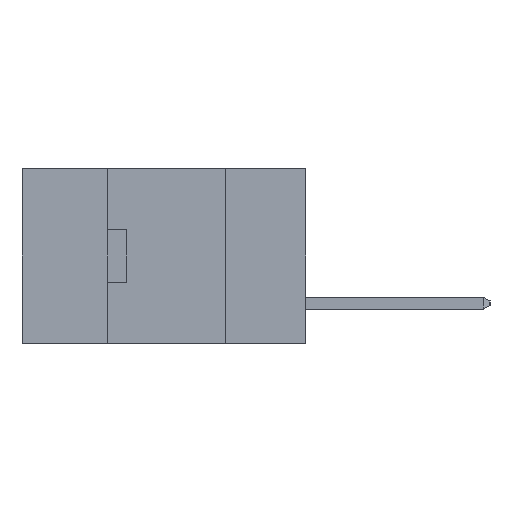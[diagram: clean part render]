
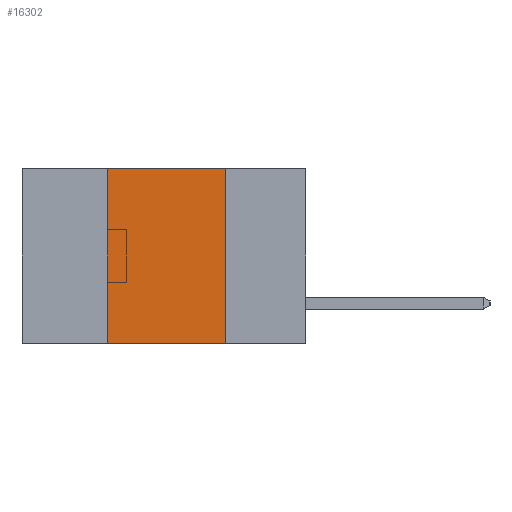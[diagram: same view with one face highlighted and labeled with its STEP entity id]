
A CAD part, left-side view. The second image highlights one B-rep face of the part: STEP entity #16302.
In plain terms, the highlighted planar face has unit normal (-1, 0, 0).
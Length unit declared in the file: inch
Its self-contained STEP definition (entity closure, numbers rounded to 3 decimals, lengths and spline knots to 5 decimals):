
#242 = ORIENTED_EDGE ( 'NONE', *, *, #8202, .F. ) ;
#1352 = PLANE ( 'NONE',  #19787 ) ;
#1804 = CARTESIAN_POINT ( 'NONE',  ( 0., 0.17, -0.37 ) ) ;
#2354 = VECTOR ( 'NONE', #24073, 39.37008 ) ;
#3273 = EDGE_CURVE ( 'NONE', #8465, #3703, #25556, .T. ) ;
#3518 = VERTEX_POINT ( 'NONE', #4085 ) ;
#3623 = DIRECTION ( 'NONE',  ( 0., 0., -1. ) ) ;
#3703 = VERTEX_POINT ( 'NONE', #25374 ) ;
#4085 = CARTESIAN_POINT ( 'NONE',  ( 0., 0.17, 0. ) ) ;
#4532 = VECTOR ( 'NONE', #14886, 39.37008 ) ;
#5842 = ORIENTED_EDGE ( 'NONE', *, *, #13503, .T. ) ;
#7167 = EDGE_LOOP ( 'NONE', ( #242, #24937, #26208, #5842 ) ) ;
#7629 = VECTOR ( 'NONE', #22485, 39.37008 ) ;
#7667 = CARTESIAN_POINT ( 'NONE',  ( 0., 0.6, 0. ) ) ;
#8202 = EDGE_CURVE ( 'NONE', #3518, #15794, #16063, .T. ) ;
#8465 = VERTEX_POINT ( 'NONE', #21970 ) ;
#10513 = CARTESIAN_POINT ( 'NONE',  ( 0., 0.17, -0.37 ) ) ;
#13503 = EDGE_CURVE ( 'NONE', #8465, #15794, #14542, .T. ) ;
#14542 = LINE ( 'NONE', #22995, #19451 ) ;
#14760 = DIRECTION ( 'NONE',  ( 0., -1., 0. ) ) ;
#14886 = DIRECTION ( 'NONE',  ( 0., 0., -1. ) ) ;
#15061 = FACE_OUTER_BOUND ( 'NONE', #7167, .T. ) ;
#15794 = VERTEX_POINT ( 'NONE', #10513 ) ;
#16063 = LINE ( 'NONE', #1804, #4532 ) ;
#16302 = ADVANCED_FACE ( 'NONE', ( #15061 ), #1352, .F. ) ;
#16573 = DIRECTION ( 'NONE',  ( 1., 0., 0. ) ) ;
#19451 = VECTOR ( 'NONE', #14760, 39.37008 ) ;
#19787 = AXIS2_PLACEMENT_3D ( 'NONE', #22699, #16573, #3623 ) ;
#21033 = EDGE_CURVE ( 'NONE', #3703, #3518, #23153, .T. ) ;
#21970 = CARTESIAN_POINT ( 'NONE',  ( 0., 0.42, -0.37 ) ) ;
#22485 = DIRECTION ( 'NONE',  ( 0., -1., 0. ) ) ;
#22699 = CARTESIAN_POINT ( 'NONE',  ( 0., 0.6, 0. ) ) ;
#22995 = CARTESIAN_POINT ( 'NONE',  ( 0., 0.6, -0.37 ) ) ;
#23153 = LINE ( 'NONE', #7667, #7629 ) ;
#24073 = DIRECTION ( 'NONE',  ( 0., 0., 1. ) ) ;
#24507 = CARTESIAN_POINT ( 'NONE',  ( 0., 0.42, -0.37 ) ) ;
#24937 = ORIENTED_EDGE ( 'NONE', *, *, #21033, .F. ) ;
#25374 = CARTESIAN_POINT ( 'NONE',  ( 0., 0.42, 0. ) ) ;
#25556 = LINE ( 'NONE', #24507, #2354 ) ;
#26208 = ORIENTED_EDGE ( 'NONE', *, *, #3273, .F. ) ;
